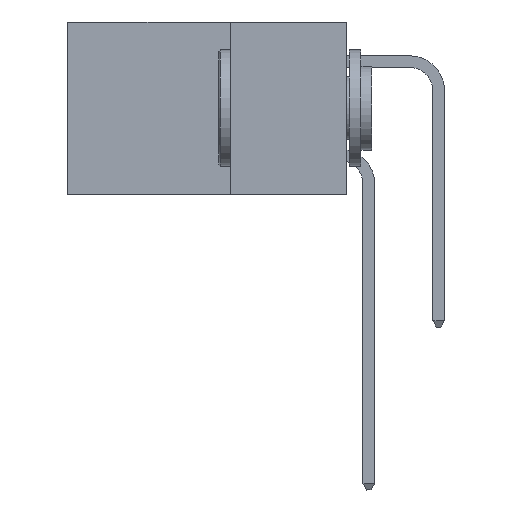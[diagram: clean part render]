
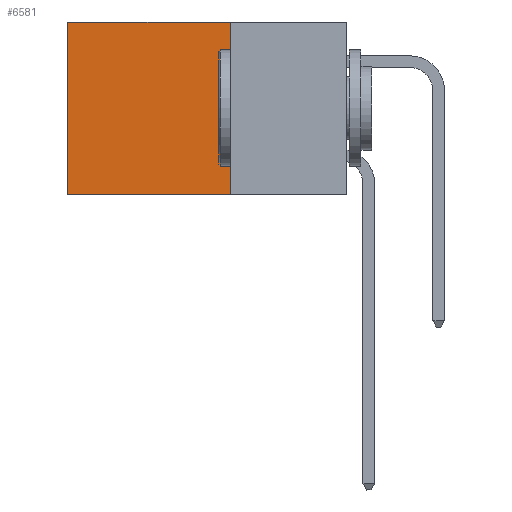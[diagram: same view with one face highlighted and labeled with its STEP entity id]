
A CAD part, left-side view. The second image highlights one B-rep face of the part: STEP entity #6581.
In plain terms, the highlighted planar face has unit normal (-1, 0, 0).
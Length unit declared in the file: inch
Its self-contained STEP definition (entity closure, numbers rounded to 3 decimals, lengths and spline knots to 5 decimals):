
#1339 = CARTESIAN_POINT ( 'NONE',  ( 0.2875, 0.25, 0. ) ) ;
#1629 = VECTOR ( 'NONE', #5919, 39.37008 ) ;
#1682 = FACE_OUTER_BOUND ( 'NONE', #15845, .T. ) ;
#2471 = VERTEX_POINT ( 'NONE', #13433 ) ;
#3066 = CARTESIAN_POINT ( 'NONE',  ( 0.2875, 0.25, 0. ) ) ;
#3334 = ORIENTED_EDGE ( 'NONE', *, *, #12138, .T. ) ;
#3555 = CARTESIAN_POINT ( 'NONE',  ( 0.2875, 0.25, 0. ) ) ;
#3748 = VERTEX_POINT ( 'NONE', #16102 ) ;
#4340 = PLANE ( 'NONE',  #11089 ) ;
#4412 = ORIENTED_EDGE ( 'NONE', *, *, #12322, .F. ) ;
#4706 = VECTOR ( 'NONE', #5470, 39.37008 ) ;
#4870 = ORIENTED_EDGE ( 'NONE', *, *, #15827, .T. ) ;
#4943 = VERTEX_POINT ( 'NONE', #8460 ) ;
#5313 = LINE ( 'NONE', #10762, #8551 ) ;
#5470 = DIRECTION ( 'NONE',  ( 0., 1., 0. ) ) ;
#5546 = LINE ( 'NONE', #3066, #1629 ) ;
#5919 = DIRECTION ( 'NONE',  ( 0., 0., -1. ) ) ;
#6581 = ADVANCED_FACE ( 'NONE', ( #1682 ), #4340, .F. ) ;
#7022 = DIRECTION ( 'NONE',  ( 0., 1., 0. ) ) ;
#7076 = CARTESIAN_POINT ( 'NONE',  ( 0.2875, 0.25, -0.37 ) ) ;
#8460 = CARTESIAN_POINT ( 'NONE',  ( 0.2875, 0.6, -0.37 ) ) ;
#8551 = VECTOR ( 'NONE', #9538, 39.37008 ) ;
#9004 = VECTOR ( 'NONE', #7022, 39.37008 ) ;
#9538 = DIRECTION ( 'NONE',  ( 0., 0., -1. ) ) ;
#9807 = CARTESIAN_POINT ( 'NONE',  ( 0.2875, 0.25, 0. ) ) ;
#10248 = DIRECTION ( 'NONE',  ( 1., 0., 0. ) ) ;
#10477 = VERTEX_POINT ( 'NONE', #3555 ) ;
#10762 = CARTESIAN_POINT ( 'NONE',  ( 0.2875, 0.6, 0. ) ) ;
#11089 = AXIS2_PLACEMENT_3D ( 'NONE', #1339, #10248, #17581 ) ;
#12138 = EDGE_CURVE ( 'NONE', #3748, #4943, #5313, .T. ) ;
#12322 = EDGE_CURVE ( 'NONE', #2471, #4943, #12882, .T. ) ;
#12463 = EDGE_CURVE ( 'NONE', #10477, #2471, #5546, .T. ) ;
#12882 = LINE ( 'NONE', #7076, #9004 ) ;
#12941 = LINE ( 'NONE', #9807, #4706 ) ;
#13294 = ORIENTED_EDGE ( 'NONE', *, *, #12463, .F. ) ;
#13433 = CARTESIAN_POINT ( 'NONE',  ( 0.2875, 0.25, -0.37 ) ) ;
#15827 = EDGE_CURVE ( 'NONE', #10477, #3748, #12941, .T. ) ;
#15845 = EDGE_LOOP ( 'NONE', ( #3334, #4412, #13294, #4870 ) ) ;
#16102 = CARTESIAN_POINT ( 'NONE',  ( 0.2875, 0.6, 0. ) ) ;
#17581 = DIRECTION ( 'NONE',  ( 0., 0., -1. ) ) ;
